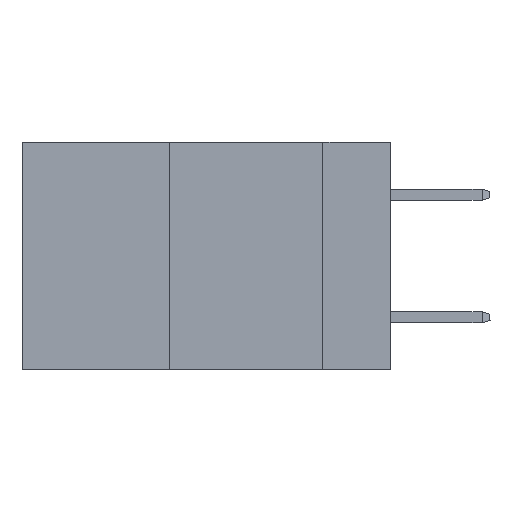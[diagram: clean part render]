
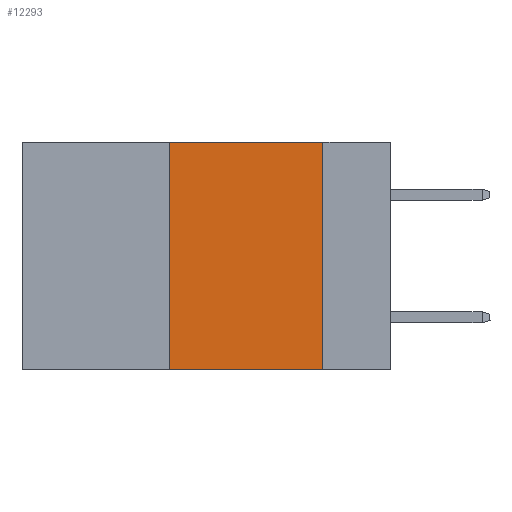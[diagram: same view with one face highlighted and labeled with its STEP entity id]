
A CAD part, left-side view. The second image highlights one B-rep face of the part: STEP entity #12293.
In plain terms, the highlighted planar face has unit normal (-1, 0, 0).
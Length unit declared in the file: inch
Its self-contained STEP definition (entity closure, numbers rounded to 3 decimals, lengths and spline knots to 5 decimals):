
#892 = EDGE_CURVE ( 'NONE', #18571, #40523, #37249, .T. ) ;
#2118 = DIRECTION ( 'NONE',  ( 1., 0., 0. ) ) ;
#4118 = VECTOR ( 'NONE', #5117, 39.37008 ) ;
#4248 = CARTESIAN_POINT ( 'NONE',  ( 0., 0.36, -0.37 ) ) ;
#4450 = VECTOR ( 'NONE', #26937, 39.37008 ) ;
#5117 = DIRECTION ( 'NONE',  ( 0., 0., 1. ) ) ;
#5193 = ORIENTED_EDGE ( 'NONE', *, *, #40682, .T. ) ;
#6794 = CARTESIAN_POINT ( 'NONE',  ( 0., 0.6, 0. ) ) ;
#6957 = EDGE_CURVE ( 'NONE', #17808, #31002, #37924, .T. ) ;
#7423 = VECTOR ( 'NONE', #21397, 39.37008 ) ;
#8142 = CARTESIAN_POINT ( 'NONE',  ( 0., 0.11, -0.37 ) ) ;
#9435 = AXIS2_PLACEMENT_3D ( 'NONE', #27011, #2118, #23897 ) ;
#12293 = ADVANCED_FACE ( 'NONE', ( #41619 ), #12414, .F. ) ;
#12414 = PLANE ( 'NONE',  #9435 ) ;
#14110 = CARTESIAN_POINT ( 'NONE',  ( 0., 0.36, 0. ) ) ;
#16374 = CARTESIAN_POINT ( 'NONE',  ( 0., 0.36, 0. ) ) ;
#17808 = VERTEX_POINT ( 'NONE', #4248 ) ;
#18571 = VERTEX_POINT ( 'NONE', #36244 ) ;
#18672 = EDGE_CURVE ( 'NONE', #31002, #18571, #39591, .T. ) ;
#19654 = ORIENTED_EDGE ( 'NONE', *, *, #892, .F. ) ;
#21397 = DIRECTION ( 'NONE',  ( 0., -1., 0. ) ) ;
#23485 = VECTOR ( 'NONE', #35192, 39.37008 ) ;
#23897 = DIRECTION ( 'NONE',  ( 0., 0., -1. ) ) ;
#25533 = ORIENTED_EDGE ( 'NONE', *, *, #6957, .F. ) ;
#26937 = DIRECTION ( 'NONE',  ( 0., 0., -1. ) ) ;
#27011 = CARTESIAN_POINT ( 'NONE',  ( 0., 0.6, 0. ) ) ;
#31002 = VERTEX_POINT ( 'NONE', #14110 ) ;
#33953 = EDGE_LOOP ( 'NONE', ( #19654, #45292, #25533, #5193 ) ) ;
#34473 = LINE ( 'NONE', #41648, #23485 ) ;
#35192 = DIRECTION ( 'NONE',  ( 0., -1., 0. ) ) ;
#36244 = CARTESIAN_POINT ( 'NONE',  ( 0., 0.11, 0. ) ) ;
#37249 = LINE ( 'NONE', #41065, #4450 ) ;
#37924 = LINE ( 'NONE', #16374, #4118 ) ;
#39591 = LINE ( 'NONE', #6794, #7423 ) ;
#40523 = VERTEX_POINT ( 'NONE', #8142 ) ;
#40682 = EDGE_CURVE ( 'NONE', #17808, #40523, #34473, .T. ) ;
#41065 = CARTESIAN_POINT ( 'NONE',  ( 0., 0.11, 0. ) ) ;
#41619 = FACE_OUTER_BOUND ( 'NONE', #33953, .T. ) ;
#41648 = CARTESIAN_POINT ( 'NONE',  ( 0., 0.6, -0.37 ) ) ;
#45292 = ORIENTED_EDGE ( 'NONE', *, *, #18672, .F. ) ;
